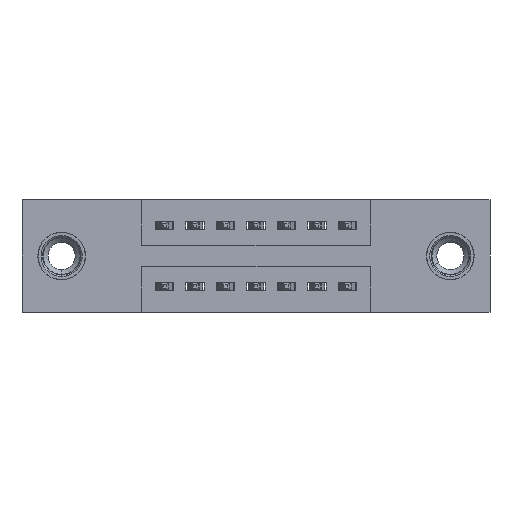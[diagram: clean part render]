
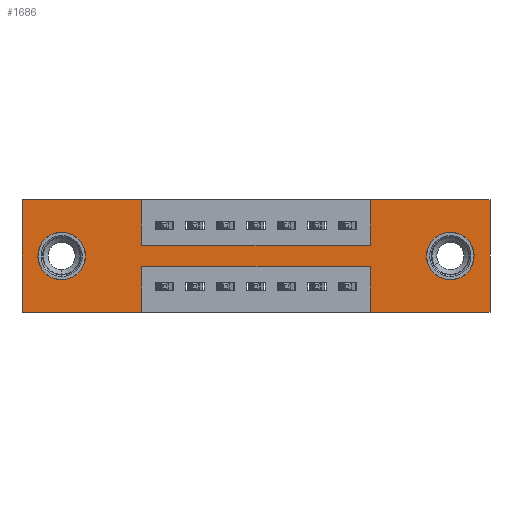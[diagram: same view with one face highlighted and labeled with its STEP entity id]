
A CAD part, front view. The second image highlights one B-rep face of the part: STEP entity #1686.
In plain terms, the highlighted planar face has unit normal (0, -1, 0).
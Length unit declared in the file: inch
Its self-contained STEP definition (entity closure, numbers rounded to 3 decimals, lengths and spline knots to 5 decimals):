
#240 = LINE ( 'NONE', #9018, #10192 ) ;
#411 = AXIS2_PLACEMENT_3D ( 'NONE', #7238, #1972, #10634 ) ;
#519 = EDGE_CURVE ( 'NONE', #8596, #6757, #3355, .T. ) ;
#565 = CARTESIAN_POINT ( 'NONE',  ( 1.535, 0., 0. ) ) ;
#671 = VERTEX_POINT ( 'NONE', #4688 ) ;
#701 = AXIS2_PLACEMENT_3D ( 'NONE', #1859, #9717, #10637 ) ;
#724 = FACE_BOUND ( 'NONE', #4218, .T. ) ;
#1017 = ORIENTED_EDGE ( 'NONE', *, *, #4201, .T. ) ;
#1021 = CARTESIAN_POINT ( 'NONE',  ( 0., 0., 0. ) ) ;
#1060 = CARTESIAN_POINT ( 'NONE',  ( 1.405, 0., -0.107 ) ) ;
#1140 = VECTOR ( 'NONE', #7507, 39.37008 ) ;
#1279 = CARTESIAN_POINT ( 'NONE',  ( 1.1425, 0., -0.37 ) ) ;
#1280 = LINE ( 'NONE', #9238, #1140 ) ;
#1343 = ORIENTED_EDGE ( 'NONE', *, *, #6693, .F. ) ;
#1420 = DIRECTION ( 'NONE',  ( 0., 0., 1. ) ) ;
#1458 = VERTEX_POINT ( 'NONE', #2718 ) ;
#1590 = ORIENTED_EDGE ( 'NONE', *, *, #8759, .F. ) ;
#1617 = VERTEX_POINT ( 'NONE', #6771 ) ;
#1686 = ADVANCED_FACE ( 'NONE', ( #724, #8408, #10501 ), #4525, .T. ) ;
#1829 = CARTESIAN_POINT ( 'NONE',  ( 0.3925, 0., -0.22 ) ) ;
#1859 = CARTESIAN_POINT ( 'NONE',  ( 0.13, 0., -0.185 ) ) ;
#1864 = CARTESIAN_POINT ( 'NONE',  ( 0., 0., 0. ) ) ;
#1883 = VECTOR ( 'NONE', #3715, 39.37008 ) ;
#1892 = ORIENTED_EDGE ( 'NONE', *, *, #2461, .F. ) ;
#1972 = DIRECTION ( 'NONE',  ( 0., 1., 0. ) ) ;
#2052 = ORIENTED_EDGE ( 'NONE', *, *, #9090, .F. ) ;
#2061 = VERTEX_POINT ( 'NONE', #5562 ) ;
#2220 = EDGE_CURVE ( 'NONE', #7092, #1617, #6633, .T. ) ;
#2241 = LINE ( 'NONE', #11106, #11343 ) ;
#2267 = CARTESIAN_POINT ( 'NONE',  ( 0.3925, 0., -0.15 ) ) ;
#2324 = VECTOR ( 'NONE', #7648, 39.37008 ) ;
#2373 = AXIS2_PLACEMENT_3D ( 'NONE', #7006, #10615, #8860 ) ;
#2461 = EDGE_CURVE ( 'NONE', #7526, #1458, #8397, .T. ) ;
#2547 = ORIENTED_EDGE ( 'NONE', *, *, #3479, .F. ) ;
#2704 = DIRECTION ( 'NONE',  ( 1., 0., 0. ) ) ;
#2705 = AXIS2_PLACEMENT_3D ( 'NONE', #3731, #5594, #3762 ) ;
#2718 = CARTESIAN_POINT ( 'NONE',  ( 1.535, 0., 0. ) ) ;
#2973 = VERTEX_POINT ( 'NONE', #7158 ) ;
#3128 = EDGE_CURVE ( 'NONE', #2973, #10384, #4063, .T. ) ;
#3141 = CARTESIAN_POINT ( 'NONE',  ( 1.1425, 0., -0.37 ) ) ;
#3150 = DIRECTION ( 'NONE',  ( 0., 0., -1. ) ) ;
#3355 = LINE ( 'NONE', #4164, #10123 ) ;
#3383 = VECTOR ( 'NONE', #4552, 39.37008 ) ;
#3392 = VERTEX_POINT ( 'NONE', #10832 ) ;
#3479 = EDGE_CURVE ( 'NONE', #6757, #4956, #6189, .T. ) ;
#3538 = ORIENTED_EDGE ( 'NONE', *, *, #2220, .F. ) ;
#3590 = EDGE_CURVE ( 'NONE', #2061, #3392, #5920, .T. ) ;
#3715 = DIRECTION ( 'NONE',  ( 1., 0., 0. ) ) ;
#3731 = CARTESIAN_POINT ( 'NONE',  ( 0.13, 0., -0.185 ) ) ;
#3745 = CIRCLE ( 'NONE', #411, 0.078 ) ;
#3762 = DIRECTION ( 'NONE',  ( 0., 0., 1. ) ) ;
#4007 = CARTESIAN_POINT ( 'NONE',  ( 1.1425, 0., -0.15 ) ) ;
#4063 = CIRCLE ( 'NONE', #2373, 0.078 ) ;
#4164 = CARTESIAN_POINT ( 'NONE',  ( 0.3925, 0., 0. ) ) ;
#4201 = EDGE_CURVE ( 'NONE', #10599, #9148, #9575, .T. ) ;
#4218 = EDGE_LOOP ( 'NONE', ( #5356, #7989 ) ) ;
#4254 = EDGE_LOOP ( 'NONE', ( #8571, #1017 ) ) ;
#4259 = VERTEX_POINT ( 'NONE', #6639 ) ;
#4525 = PLANE ( 'NONE',  #6966 ) ;
#4552 = DIRECTION ( 'NONE',  ( -1., 0., 0. ) ) ;
#4589 = ORIENTED_EDGE ( 'NONE', *, *, #5042, .F. ) ;
#4656 = LINE ( 'NONE', #8070, #1883 ) ;
#4688 = CARTESIAN_POINT ( 'NONE',  ( 0.3925, 0., -0.37 ) ) ;
#4694 = CARTESIAN_POINT ( 'NONE',  ( 1.1425, 0., 0. ) ) ;
#4829 = VECTOR ( 'NONE', #1420, 39.37008 ) ;
#4854 = VECTOR ( 'NONE', #3150, 39.37008 ) ;
#4891 = DIRECTION ( 'NONE',  ( 0., 0., -1. ) ) ;
#4956 = VERTEX_POINT ( 'NONE', #4007 ) ;
#4967 = DIRECTION ( 'NONE',  ( -1., 0., 0. ) ) ;
#5042 = EDGE_CURVE ( 'NONE', #3392, #671, #2241, .T. ) ;
#5321 = EDGE_CURVE ( 'NONE', #10384, #2973, #3745, .T. ) ;
#5356 = ORIENTED_EDGE ( 'NONE', *, *, #5321, .T. ) ;
#5427 = EDGE_CURVE ( 'NONE', #671, #7092, #1280, .T. ) ;
#5562 = CARTESIAN_POINT ( 'NONE',  ( 1.1425, 0., -0.22 ) ) ;
#5594 = DIRECTION ( 'NONE',  ( 0., 1., 0. ) ) ;
#5916 = DIRECTION ( 'NONE',  ( 1., 0., 0. ) ) ;
#5920 = LINE ( 'NONE', #1829, #3383 ) ;
#6035 = EDGE_LOOP ( 'NONE', ( #4589, #8643, #2052, #10443, #1343, #1892, #9469, #2547, #6788, #1590, #3538, #8461 ) ) ;
#6187 = EDGE_CURVE ( 'NONE', #9148, #10599, #7180, .T. ) ;
#6189 = LINE ( 'NONE', #2267, #9733 ) ;
#6222 = LINE ( 'NONE', #10208, #6627 ) ;
#6627 = VECTOR ( 'NONE', #4967, 39.37008 ) ;
#6633 = LINE ( 'NONE', #1021, #4829 ) ;
#6639 = CARTESIAN_POINT ( 'NONE',  ( 1.535, 0., -0.37 ) ) ;
#6693 = EDGE_CURVE ( 'NONE', #1458, #4259, #9921, .T. ) ;
#6757 = VERTEX_POINT ( 'NONE', #8685 ) ;
#6771 = CARTESIAN_POINT ( 'NONE',  ( 0., 0., 0. ) ) ;
#6788 = ORIENTED_EDGE ( 'NONE', *, *, #519, .F. ) ;
#6966 = AXIS2_PLACEMENT_3D ( 'NONE', #11432, #10660, #9695 ) ;
#7006 = CARTESIAN_POINT ( 'NONE',  ( 1.405, 0., -0.185 ) ) ;
#7010 = CARTESIAN_POINT ( 'NONE',  ( 0.3925, 0., 0. ) ) ;
#7028 = CARTESIAN_POINT ( 'NONE',  ( 0.13, 0., -0.107 ) ) ;
#7092 = VERTEX_POINT ( 'NONE', #8697 ) ;
#7158 = CARTESIAN_POINT ( 'NONE',  ( 1.405, 0., -0.263 ) ) ;
#7180 = CIRCLE ( 'NONE', #2705, 0.078 ) ;
#7238 = CARTESIAN_POINT ( 'NONE',  ( 1.405, 0., -0.185 ) ) ;
#7417 = EDGE_CURVE ( 'NONE', #4956, #7526, #240, .T. ) ;
#7507 = DIRECTION ( 'NONE',  ( -1., 0., 0. ) ) ;
#7526 = VERTEX_POINT ( 'NONE', #4694 ) ;
#7602 = DIRECTION ( 'NONE',  ( 0., 0., -1. ) ) ;
#7648 = DIRECTION ( 'NONE',  ( 0., 0., 1. ) ) ;
#7765 = EDGE_CURVE ( 'NONE', #4259, #9486, #6222, .T. ) ;
#7989 = ORIENTED_EDGE ( 'NONE', *, *, #3128, .T. ) ;
#8013 = VECTOR ( 'NONE', #2704, 39.37008 ) ;
#8027 = CARTESIAN_POINT ( 'NONE',  ( 0.13, 0., -0.263 ) ) ;
#8070 = CARTESIAN_POINT ( 'NONE',  ( 0., 0., 0. ) ) ;
#8397 = LINE ( 'NONE', #1864, #8013 ) ;
#8408 = FACE_BOUND ( 'NONE', #4254, .T. ) ;
#8461 = ORIENTED_EDGE ( 'NONE', *, *, #5427, .F. ) ;
#8571 = ORIENTED_EDGE ( 'NONE', *, *, #6187, .T. ) ;
#8596 = VERTEX_POINT ( 'NONE', #7010 ) ;
#8643 = ORIENTED_EDGE ( 'NONE', *, *, #3590, .F. ) ;
#8685 = CARTESIAN_POINT ( 'NONE',  ( 0.3925, 0., -0.15 ) ) ;
#8697 = CARTESIAN_POINT ( 'NONE',  ( 0., 0., -0.37 ) ) ;
#8759 = EDGE_CURVE ( 'NONE', #1617, #8596, #4656, .T. ) ;
#8860 = DIRECTION ( 'NONE',  ( 0., 0., -1. ) ) ;
#9018 = CARTESIAN_POINT ( 'NONE',  ( 1.1425, 0., 0. ) ) ;
#9090 = EDGE_CURVE ( 'NONE', #9486, #2061, #9780, .T. ) ;
#9148 = VERTEX_POINT ( 'NONE', #7028 ) ;
#9238 = CARTESIAN_POINT ( 'NONE',  ( 0., 0., -0.37 ) ) ;
#9469 = ORIENTED_EDGE ( 'NONE', *, *, #7417, .F. ) ;
#9486 = VERTEX_POINT ( 'NONE', #1279 ) ;
#9575 = CIRCLE ( 'NONE', #701, 0.078 ) ;
#9695 = DIRECTION ( 'NONE',  ( 0., 0., -1. ) ) ;
#9717 = DIRECTION ( 'NONE',  ( 0., 1., 0. ) ) ;
#9733 = VECTOR ( 'NONE', #5916, 39.37008 ) ;
#9780 = LINE ( 'NONE', #3141, #2324 ) ;
#9921 = LINE ( 'NONE', #565, #4854 ) ;
#10123 = VECTOR ( 'NONE', #7602, 39.37008 ) ;
#10192 = VECTOR ( 'NONE', #10809, 39.37008 ) ;
#10208 = CARTESIAN_POINT ( 'NONE',  ( 0., 0., -0.37 ) ) ;
#10384 = VERTEX_POINT ( 'NONE', #1060 ) ;
#10443 = ORIENTED_EDGE ( 'NONE', *, *, #7765, .F. ) ;
#10501 = FACE_OUTER_BOUND ( 'NONE', #6035, .T. ) ;
#10599 = VERTEX_POINT ( 'NONE', #8027 ) ;
#10615 = DIRECTION ( 'NONE',  ( 0., 1., 0. ) ) ;
#10634 = DIRECTION ( 'NONE',  ( 0., 0., -1. ) ) ;
#10637 = DIRECTION ( 'NONE',  ( 0., 0., 1. ) ) ;
#10660 = DIRECTION ( 'NONE',  ( 0., -1., 0. ) ) ;
#10809 = DIRECTION ( 'NONE',  ( 0., 0., 1. ) ) ;
#10832 = CARTESIAN_POINT ( 'NONE',  ( 0.3925, 0., -0.22 ) ) ;
#11106 = CARTESIAN_POINT ( 'NONE',  ( 0.3925, 0., -0.37 ) ) ;
#11343 = VECTOR ( 'NONE', #4891, 39.37008 ) ;
#11432 = CARTESIAN_POINT ( 'NONE',  ( 0., 0., -0.37 ) ) ;
